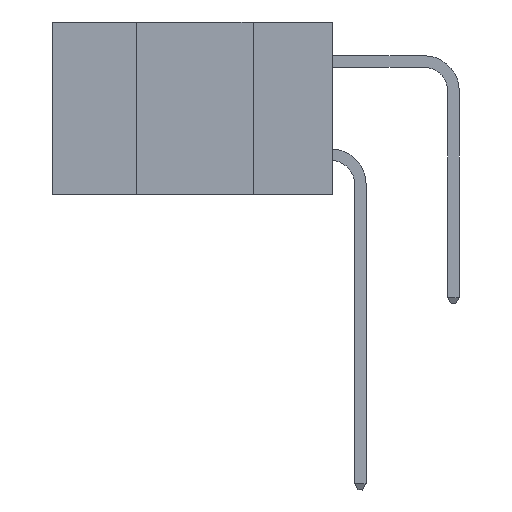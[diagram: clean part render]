
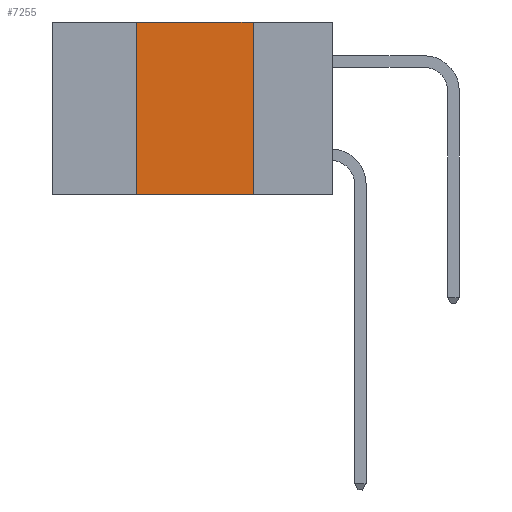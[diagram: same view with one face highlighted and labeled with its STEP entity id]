
A CAD part, left-side view. The second image highlights one B-rep face of the part: STEP entity #7255.
In plain terms, the highlighted planar face has unit normal (-1, 0, 0).
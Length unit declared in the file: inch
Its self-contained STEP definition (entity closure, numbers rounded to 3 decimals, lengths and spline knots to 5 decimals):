
#1319 = VERTEX_POINT ( 'NONE', #8238 ) ;
#2879 = ORIENTED_EDGE ( 'NONE', *, *, #14357, .F. ) ;
#3714 = DIRECTION ( 'NONE',  ( 0., -1., 0. ) ) ;
#4889 = LINE ( 'NONE', #22862, #15837 ) ;
#7255 = ADVANCED_FACE ( 'NONE', ( #15067 ), #20999, .F. ) ;
#7974 = CARTESIAN_POINT ( 'NONE',  ( 0., 0.17, -0.37 ) ) ;
#8238 = CARTESIAN_POINT ( 'NONE',  ( 0., 0.17, 0. ) ) ;
#9121 = VECTOR ( 'NONE', #16321, 39.37008 ) ;
#9479 = CARTESIAN_POINT ( 'NONE',  ( 0., 0.6, 0. ) ) ;
#9568 = VERTEX_POINT ( 'NONE', #22550 ) ;
#10210 = ORIENTED_EDGE ( 'NONE', *, *, #11783, .T. ) ;
#10780 = AXIS2_PLACEMENT_3D ( 'NONE', #9479, #11439, #24843 ) ;
#11158 = ORIENTED_EDGE ( 'NONE', *, *, #24635, .F. ) ;
#11439 = DIRECTION ( 'NONE',  ( 1., 0., 0. ) ) ;
#11783 = EDGE_CURVE ( 'NONE', #11909, #9568, #4889, .T. ) ;
#11909 = VERTEX_POINT ( 'NONE', #17585 ) ;
#11910 = DIRECTION ( 'NONE',  ( 0., 0., -1. ) ) ;
#12223 = DIRECTION ( 'NONE',  ( 0., -1., 0. ) ) ;
#13831 = VECTOR ( 'NONE', #11910, 39.37008 ) ;
#13967 = EDGE_LOOP ( 'NONE', ( #11158, #18361, #2879, #10210 ) ) ;
#14357 = EDGE_CURVE ( 'NONE', #11909, #23206, #24457, .T. ) ;
#14380 = CARTESIAN_POINT ( 'NONE',  ( 0., 0.42, -0.37 ) ) ;
#15067 = FACE_OUTER_BOUND ( 'NONE', #13967, .T. ) ;
#15105 = VECTOR ( 'NONE', #12223, 39.37008 ) ;
#15837 = VECTOR ( 'NONE', #3714, 39.37008 ) ;
#16321 = DIRECTION ( 'NONE',  ( 0., 0., 1. ) ) ;
#17444 = CARTESIAN_POINT ( 'NONE',  ( 0., 0.42, 0. ) ) ;
#17585 = CARTESIAN_POINT ( 'NONE',  ( 0., 0.42, -0.37 ) ) ;
#17949 = CARTESIAN_POINT ( 'NONE',  ( 0., 0.6, 0. ) ) ;
#18361 = ORIENTED_EDGE ( 'NONE', *, *, #20793, .F. ) ;
#18942 = LINE ( 'NONE', #7974, #13831 ) ;
#20793 = EDGE_CURVE ( 'NONE', #23206, #1319, #24673, .T. ) ;
#20999 = PLANE ( 'NONE',  #10780 ) ;
#22550 = CARTESIAN_POINT ( 'NONE',  ( 0., 0.17, -0.37 ) ) ;
#22862 = CARTESIAN_POINT ( 'NONE',  ( 0., 0.6, -0.37 ) ) ;
#23206 = VERTEX_POINT ( 'NONE', #17444 ) ;
#24457 = LINE ( 'NONE', #14380, #9121 ) ;
#24635 = EDGE_CURVE ( 'NONE', #1319, #9568, #18942, .T. ) ;
#24673 = LINE ( 'NONE', #17949, #15105 ) ;
#24843 = DIRECTION ( 'NONE',  ( 0., 0., -1. ) ) ;
